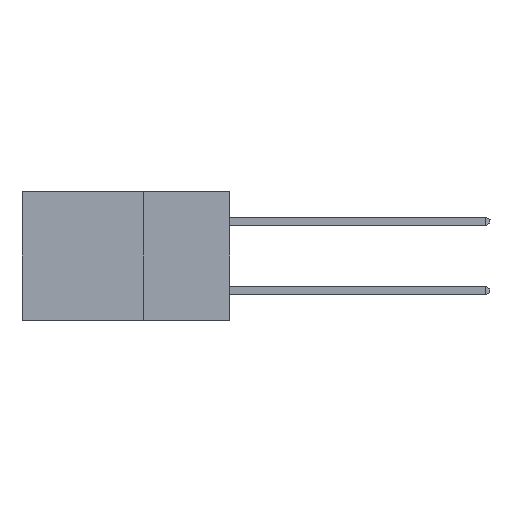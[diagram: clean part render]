
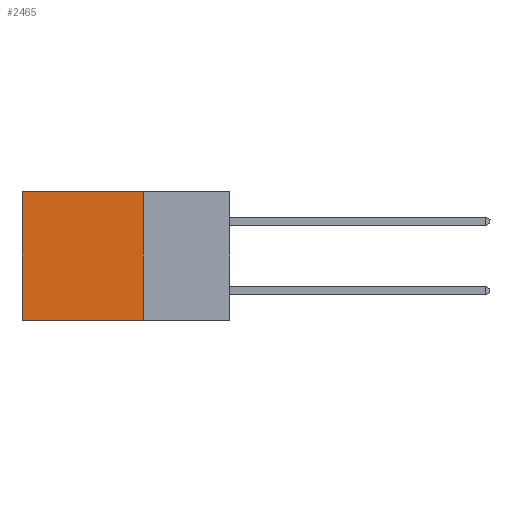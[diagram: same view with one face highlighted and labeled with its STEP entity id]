
A CAD part, left-side view. The second image highlights one B-rep face of the part: STEP entity #2465.
In plain terms, the highlighted planar face has unit normal (-1, 0, 0).
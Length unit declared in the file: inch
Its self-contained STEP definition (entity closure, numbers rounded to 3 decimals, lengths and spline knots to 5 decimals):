
#1994 = CARTESIAN_POINT ( 'NONE',  ( 0.298, 0.25, 0. ) ) ;
#2044 = DIRECTION ( 'NONE',  ( 1., 0., 0. ) ) ;
#2465 = ADVANCED_FACE ( 'NONE', ( #9799 ), #11836, .F. ) ;
#4351 = CARTESIAN_POINT ( 'NONE',  ( 0.298, 0.25, -0.37 ) ) ;
#4828 = CARTESIAN_POINT ( 'NONE',  ( 0.298, 0.25, 0. ) ) ;
#6047 = LINE ( 'NONE', #8559, #27296 ) ;
#8559 = CARTESIAN_POINT ( 'NONE',  ( 0.298, 0.6, 0. ) ) ;
#9156 = EDGE_CURVE ( 'NONE', #20746, #17416, #24871, .T. ) ;
#9596 = VERTEX_POINT ( 'NONE', #24630 ) ;
#9799 = FACE_OUTER_BOUND ( 'NONE', #12654, .T. ) ;
#11716 = VECTOR ( 'NONE', #21270, 39.37008 ) ;
#11836 = PLANE ( 'NONE',  #12756 ) ;
#12654 = EDGE_LOOP ( 'NONE', ( #20650, #26860, #23193, #30401 ) ) ;
#12756 = AXIS2_PLACEMENT_3D ( 'NONE', #16800, #2044, #19271 ) ;
#15206 = LINE ( 'NONE', #31144, #11716 ) ;
#16568 = LINE ( 'NONE', #4351, #19642 ) ;
#16800 = CARTESIAN_POINT ( 'NONE',  ( 0.298, 0.25, 0. ) ) ;
#17416 = VERTEX_POINT ( 'NONE', #27644 ) ;
#18168 = VERTEX_POINT ( 'NONE', #30883 ) ;
#18353 = DIRECTION ( 'NONE',  ( 0., 0., -1. ) ) ;
#18495 = EDGE_CURVE ( 'NONE', #17416, #9596, #6047, .T. ) ;
#19271 = DIRECTION ( 'NONE',  ( 0., 0., -1. ) ) ;
#19642 = VECTOR ( 'NONE', #26496, 39.37008 ) ;
#20650 = ORIENTED_EDGE ( 'NONE', *, *, #18495, .T. ) ;
#20746 = VERTEX_POINT ( 'NONE', #1994 ) ;
#21270 = DIRECTION ( 'NONE',  ( 0., 0., -1. ) ) ;
#22927 = EDGE_CURVE ( 'NONE', #18168, #9596, #16568, .T. ) ;
#22937 = VECTOR ( 'NONE', #27190, 39.37008 ) ;
#23193 = ORIENTED_EDGE ( 'NONE', *, *, #29761, .F. ) ;
#24630 = CARTESIAN_POINT ( 'NONE',  ( 0.298, 0.6, -0.37 ) ) ;
#24871 = LINE ( 'NONE', #4828, #22937 ) ;
#26496 = DIRECTION ( 'NONE',  ( 0., 1., 0. ) ) ;
#26860 = ORIENTED_EDGE ( 'NONE', *, *, #22927, .F. ) ;
#27190 = DIRECTION ( 'NONE',  ( 0., 1., 0. ) ) ;
#27296 = VECTOR ( 'NONE', #18353, 39.37008 ) ;
#27644 = CARTESIAN_POINT ( 'NONE',  ( 0.298, 0.6, 0. ) ) ;
#29761 = EDGE_CURVE ( 'NONE', #20746, #18168, #15206, .T. ) ;
#30401 = ORIENTED_EDGE ( 'NONE', *, *, #9156, .T. ) ;
#30883 = CARTESIAN_POINT ( 'NONE',  ( 0.298, 0.25, -0.37 ) ) ;
#31144 = CARTESIAN_POINT ( 'NONE',  ( 0.298, 0.25, 0. ) ) ;
